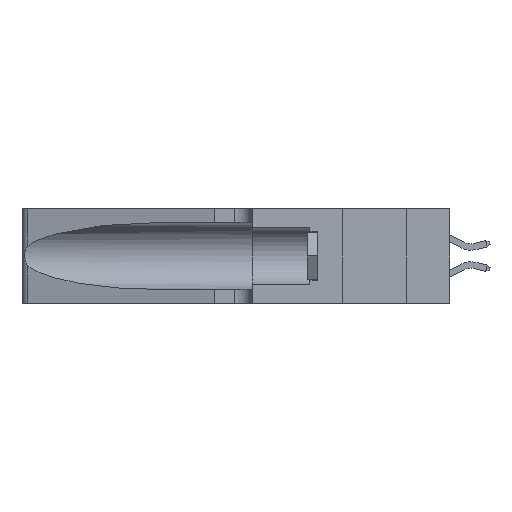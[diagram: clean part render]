
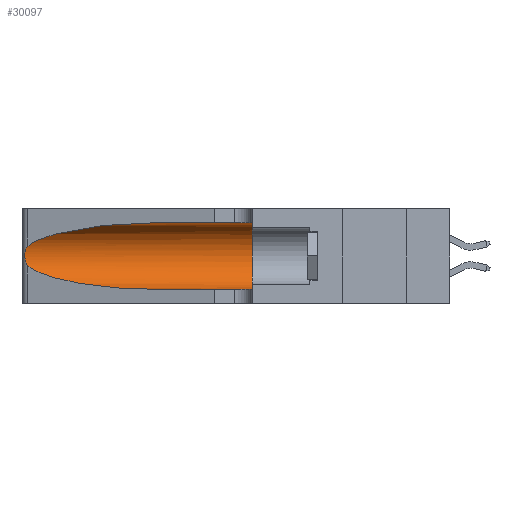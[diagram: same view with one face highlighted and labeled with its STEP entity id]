
A CAD part, left-side view. The second image highlights one B-rep face of the part: STEP entity #30097.
In plain terms, the highlighted cylindrical face has radius 3.308 mm (diameter 6.617 mm), a partial arc.
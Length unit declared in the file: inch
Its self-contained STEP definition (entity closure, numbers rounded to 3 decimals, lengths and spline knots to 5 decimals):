
#959 = DIRECTION ( 'NONE',  ( 0., 0., -1. ) ) ;
#2039 = LINE ( 'NONE', #24928, #15788 ) ;
#2419 = LINE ( 'NONE', #18352, #3446 ) ;
#2948 = EDGE_CURVE ( 'NONE', #15966, #18180, #17928, .T. ) ;
#3446 = VECTOR ( 'NONE', #14534, 39.37008 ) ;
#3854 = EDGE_LOOP ( 'NONE', ( #5570, #17845, #18905, #6507, #21155, #5814 ) ) ;
#5136 = VERTEX_POINT ( 'NONE', #20577 ) ;
#5570 = ORIENTED_EDGE ( 'NONE', *, *, #25004, .T. ) ;
#5762 = CARTESIAN_POINT ( 'NONE',  ( 0.26018, 1.23835, 0.19895 ) ) ;
#5814 = ORIENTED_EDGE ( 'NONE', *, *, #19448, .F. ) ;
#5904 = CARTESIAN_POINT ( 'NONE',  ( 0.25854, 1.2359, 0.20912 ) ) ;
#6293 = FACE_OUTER_BOUND ( 'NONE', #3854, .T. ) ;
#6507 = ORIENTED_EDGE ( 'NONE', *, *, #27670, .T. ) ;
#6783 = CARTESIAN_POINT ( 'NONE',  ( 0.25487, 1.22718, 0.22369 ) ) ;
#7210 =( BOUNDED_CURVE ( )  B_SPLINE_CURVE ( 3, ( #26027, #32430, #13089, #19933 ),
 .UNSPECIFIED., .F., .F. ) 
 B_SPLINE_CURVE_WITH_KNOTS ( ( 4, 4 ),
 ( 3.44316, 4.71239 ),
 .UNSPECIFIED. ) 
 CURVE ( )  GEOMETRIC_REPRESENTATION_ITEM ( )  RATIONAL_B_SPLINE_CURVE ( ( 1., 0.87, 0.87, 1. ) ) 
 REPRESENTATION_ITEM ( '' )  );
#7499 = DIRECTION ( 'NONE',  ( 0., 1., 0. ) ) ;
#9293 = CARTESIAN_POINT ( 'NONE',  ( 0.25487, 1.22718, 0.14631 ) ) ;
#12278 = CARTESIAN_POINT ( 'NONE',  ( 0.25639, 1.23184, 0.21858 ) ) ;
#12562 = CARTESIAN_POINT ( 'NONE',  ( 0.26075, 1.23896, 0.19203 ) ) ;
#13010 = CARTESIAN_POINT ( 'NONE',  ( 0.1305, 0.35, 0.05475 ) ) ;
#13089 = CARTESIAN_POINT ( 'NONE',  ( 0.18966, 0.96281, 0.05475 ) ) ;
#14534 = DIRECTION ( 'NONE',  ( 0., -1., 0. ) ) ;
#14975 = CYLINDRICAL_SURFACE ( 'NONE', #26216, 0.13025 ) ;
#15788 = VECTOR ( 'NONE', #28193, 39.37008 ) ;
#15966 = VERTEX_POINT ( 'NONE', #25944 ) ;
#17845 = ORIENTED_EDGE ( 'NONE', *, *, #2948, .T. ) ;
#17928 = B_SPLINE_CURVE_WITH_KNOTS ( 'NONE', 3,
 ( #21304, #28087, #12278, #38122, #5904, #5762, #12562, #28774, #18857, #38406, #25515, #24962, #31900, #34862 ),
 .UNSPECIFIED., .F., .F.,
 ( 4, 2, 2, 2, 2, 2, 4 ),
 ( 0., 0.00027, 0.00053, 0.00107, 0.0016, 0.00187, 0.00214 ),
 .UNSPECIFIED. ) ;
#18180 = VERTEX_POINT ( 'NONE', #9293 ) ;
#18352 = CARTESIAN_POINT ( 'NONE',  ( 0.1305, 1.61858, 0.05475 ) ) ;
#18857 = CARTESIAN_POINT ( 'NONE',  ( 0.26017, 1.23833, 0.17102 ) ) ;
#18905 = ORIENTED_EDGE ( 'NONE', *, *, #29294, .T. ) ;
#19448 = EDGE_CURVE ( 'NONE', #41951, #28531, #2039, .T. ) ;
#19713 = CARTESIAN_POINT ( 'NONE',  ( 0.1305, 0.35, 0.31525 ) ) ;
#19933 = CARTESIAN_POINT ( 'NONE',  ( 0.1305, 0.72297, 0.05475 ) ) ;
#20577 = CARTESIAN_POINT ( 'NONE',  ( 0.1305, 0.72297, 0.05475 ) ) ;
#21155 = ORIENTED_EDGE ( 'NONE', *, *, #31454, .F. ) ;
#21304 = CARTESIAN_POINT ( 'NONE',  ( 0.25487, 1.22718, 0.22369 ) ) ;
#22735 = CARTESIAN_POINT ( 'NONE',  ( 0.18966, 0.96281, 0.31525 ) ) ;
#24928 = CARTESIAN_POINT ( 'NONE',  ( 0.1305, 1.61858, 0.31525 ) ) ;
#24962 = CARTESIAN_POINT ( 'NONE',  ( 0.25639, 1.23186, 0.15144 ) ) ;
#25004 = EDGE_CURVE ( 'NONE', #41951, #15966, #28073, .T. ) ;
#25515 = CARTESIAN_POINT ( 'NONE',  ( 0.25789, 1.23486, 0.15765 ) ) ;
#25944 = CARTESIAN_POINT ( 'NONE',  ( 0.25487, 1.22718, 0.22369 ) ) ;
#26027 = CARTESIAN_POINT ( 'NONE',  ( 0.25487, 1.22718, 0.14631 ) ) ;
#26216 = AXIS2_PLACEMENT_3D ( 'NONE', #33780, #37039, #959 ) ;
#26435 = CIRCLE ( 'NONE', #35500, 0.13025 ) ;
#26946 = CARTESIAN_POINT ( 'NONE',  ( 0.1305, 0.35, 0.185 ) ) ;
#27475 = CARTESIAN_POINT ( 'NONE',  ( 0.1305, 0.72297, 0.31525 ) ) ;
#27670 = EDGE_CURVE ( 'NONE', #5136, #39064, #2419, .T. ) ;
#28073 =( BOUNDED_CURVE ( )  B_SPLINE_CURVE ( 3, ( #41877, #22735, #32100, #6783 ),
 .UNSPECIFIED., .F., .T. ) 
 B_SPLINE_CURVE_WITH_KNOTS ( ( 4, 4 ),
 ( 1.5708, 2.84003 ),
 .UNSPECIFIED. ) 
 CURVE ( )  GEOMETRIC_REPRESENTATION_ITEM ( )  RATIONAL_B_SPLINE_CURVE ( ( 1., 0.87, 0.87, 1. ) ) 
 REPRESENTATION_ITEM ( '' )  );
#28087 = CARTESIAN_POINT ( 'NONE',  ( 0.25555, 1.22994, 0.2215 ) ) ;
#28193 = DIRECTION ( 'NONE',  ( 0., -1., 0. ) ) ;
#28531 = VERTEX_POINT ( 'NONE', #19713 ) ;
#28774 = CARTESIAN_POINT ( 'NONE',  ( 0.26075, 1.23896, 0.178 ) ) ;
#29294 = EDGE_CURVE ( 'NONE', #18180, #5136, #7210, .T. ) ;
#30097 = ADVANCED_FACE ( 'NONE', ( #6293 ), #14975, .F. ) ;
#30221 = DIRECTION ( 'NONE',  ( 0., 0., 1. ) ) ;
#31454 = EDGE_CURVE ( 'NONE', #28531, #39064, #26435, .T. ) ;
#31900 = CARTESIAN_POINT ( 'NONE',  ( 0.25555, 1.22993, 0.14849 ) ) ;
#32100 = CARTESIAN_POINT ( 'NONE',  ( 0.2373, 1.15595, 0.28018 ) ) ;
#32430 = CARTESIAN_POINT ( 'NONE',  ( 0.2373, 1.15595, 0.08982 ) ) ;
#33780 = CARTESIAN_POINT ( 'NONE',  ( 0.1305, 1.61858, 0.185 ) ) ;
#34862 = CARTESIAN_POINT ( 'NONE',  ( 0.25487, 1.22718, 0.14631 ) ) ;
#35500 = AXIS2_PLACEMENT_3D ( 'NONE', #26946, #7499, #30221 ) ;
#37039 = DIRECTION ( 'NONE',  ( 0., -1., 0. ) ) ;
#38122 = CARTESIAN_POINT ( 'NONE',  ( 0.25787, 1.23484, 0.2124 ) ) ;
#38406 = CARTESIAN_POINT ( 'NONE',  ( 0.25856, 1.23593, 0.16098 ) ) ;
#39064 = VERTEX_POINT ( 'NONE', #13010 ) ;
#41877 = CARTESIAN_POINT ( 'NONE',  ( 0.1305, 0.72297, 0.31525 ) ) ;
#41951 = VERTEX_POINT ( 'NONE', #27475 ) ;
